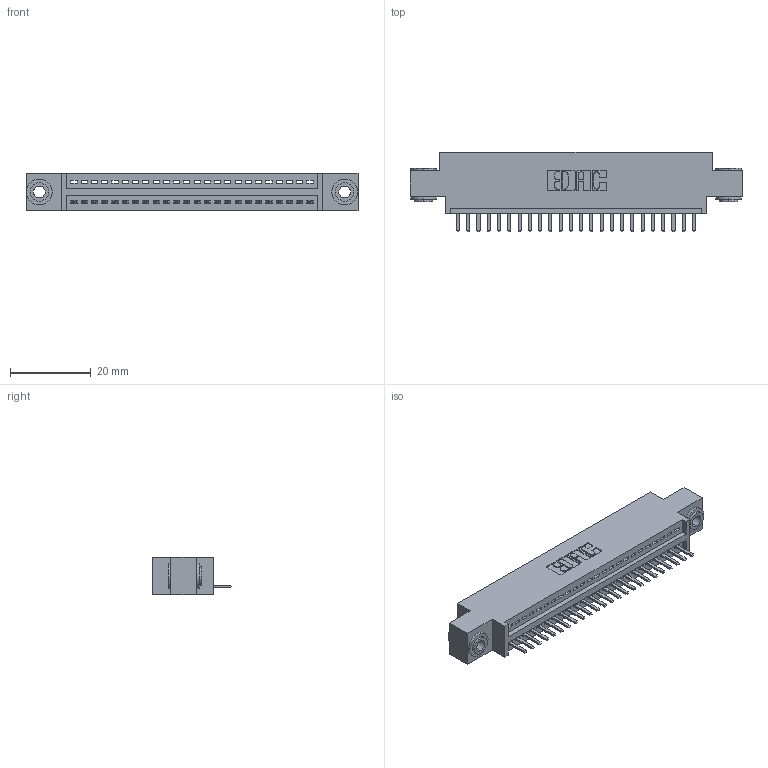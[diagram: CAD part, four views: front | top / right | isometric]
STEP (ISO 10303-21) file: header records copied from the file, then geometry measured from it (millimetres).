
FILE_DESCRIPTION (( 'STEP AP203' ), '1' );
FILE_NAME ('395-024-520-603.STEP', '2018-11-08T15:12:22', ( '' ), ( '' ), 'SwSTEP 2.0', 'SolidWorks 2016', '' );
FILE_SCHEMA (( 'CONFIG_CONTROL_DESIGN' ));
Length unit declared in the file: inch
Products named in the file (4): 345-292-001_345-293-120; 345 Part_0.170 Offset - 0.156 Dia-TH; 395-024-520-603; 345-250-002_345-250-002-102
Assembly tree (27 placements, depth 2):
  395-024-520-603
    345 Part_0.170 Offset - 0.156 Dia-TH
    345-292-001_345-293-120  x24
    345-250-002_345-250-002-102  x2
Bounding box: 82.17 x 19.68 x 9.4 mm (x, y, z)
Volume: 7494 mm3; surface area: 9829.4 mm2
Topology: 27 solids, 27 shells, 1656 faces, 4845 edges, 3162 vertices
Faces by surface type: plane 1102, cylinder 546, cone 8
Entity records: 21382 total; most frequent: CARTESIAN_POINT 3695, ORIENTED_EDGE 3634, DIRECTION 3271, EDGE_CURVE 1817, VECTOR 1561, LINE 1561, VERTEX_POINT 1206, AXIS2_PLACEMENT_3D 855
